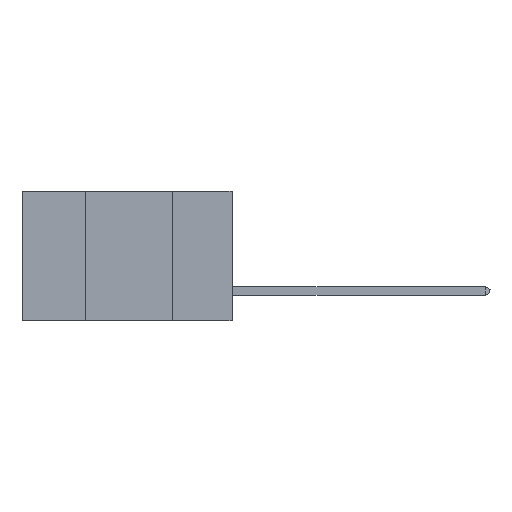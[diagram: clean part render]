
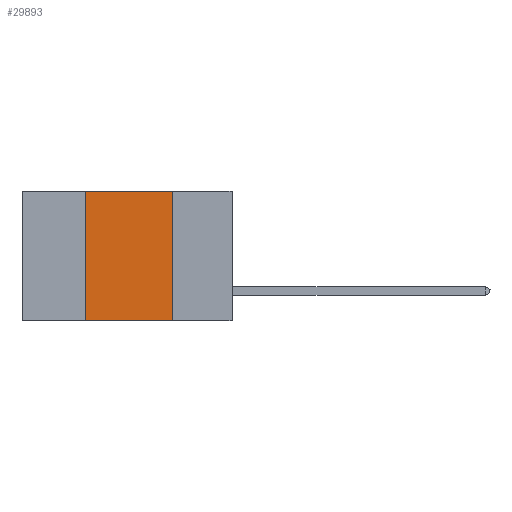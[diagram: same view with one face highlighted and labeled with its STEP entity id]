
A CAD part, left-side view. The second image highlights one B-rep face of the part: STEP entity #29893.
In plain terms, the highlighted planar face has unit normal (-1, 0, 0).
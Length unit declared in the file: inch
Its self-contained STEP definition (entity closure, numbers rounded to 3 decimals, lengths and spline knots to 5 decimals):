
#65 = EDGE_LOOP ( 'NONE', ( #20425, #28894, #29847, #20932 ) ) ;
#363 = EDGE_CURVE ( 'NONE', #22972, #16654, #29425, .T. ) ;
#664 = PLANE ( 'NONE',  #15403 ) ;
#749 = EDGE_CURVE ( 'NONE', #7456, #1954, #1974, .T. ) ;
#1749 = EDGE_CURVE ( 'NONE', #7456, #22972, #27541, .T. ) ;
#1954 = VERTEX_POINT ( 'NONE', #15884 ) ;
#1974 = LINE ( 'NONE', #10816, #25741 ) ;
#3836 = DIRECTION ( 'NONE',  ( 0., 0., 1. ) ) ;
#4505 = DIRECTION ( 'NONE',  ( 0., -1., 0. ) ) ;
#6804 = CARTESIAN_POINT ( 'NONE',  ( 0., 0.6, 0. ) ) ;
#7126 = LINE ( 'NONE', #12004, #9635 ) ;
#7456 = VERTEX_POINT ( 'NONE', #26695 ) ;
#8820 = DIRECTION ( 'NONE',  ( 0., -1., 0. ) ) ;
#9635 = VECTOR ( 'NONE', #14418, 39.37008 ) ;
#10238 = CARTESIAN_POINT ( 'NONE',  ( 0., 0.42, 0. ) ) ;
#10816 = CARTESIAN_POINT ( 'NONE',  ( 0., 0.6, -0.37 ) ) ;
#12004 = CARTESIAN_POINT ( 'NONE',  ( 0., 0.17, 0. ) ) ;
#14028 = EDGE_CURVE ( 'NONE', #16654, #1954, #7126, .T. ) ;
#14418 = DIRECTION ( 'NONE',  ( 0., 0., -1. ) ) ;
#15403 = AXIS2_PLACEMENT_3D ( 'NONE', #23320, #21112, #16593 ) ;
#15884 = CARTESIAN_POINT ( 'NONE',  ( 0., 0.17, -0.37 ) ) ;
#16593 = DIRECTION ( 'NONE',  ( 0., 0., -1. ) ) ;
#16654 = VERTEX_POINT ( 'NONE', #18955 ) ;
#17511 = VECTOR ( 'NONE', #4505, 39.37008 ) ;
#17647 = CARTESIAN_POINT ( 'NONE',  ( 0., 0.42, 0. ) ) ;
#18955 = CARTESIAN_POINT ( 'NONE',  ( 0., 0.17, 0. ) ) ;
#20425 = ORIENTED_EDGE ( 'NONE', *, *, #14028, .F. ) ;
#20932 = ORIENTED_EDGE ( 'NONE', *, *, #749, .T. ) ;
#21112 = DIRECTION ( 'NONE',  ( 1., 0., 0. ) ) ;
#22972 = VERTEX_POINT ( 'NONE', #10238 ) ;
#23320 = CARTESIAN_POINT ( 'NONE',  ( 0., 0.6, 0. ) ) ;
#23782 = FACE_OUTER_BOUND ( 'NONE', #65, .T. ) ;
#23875 = VECTOR ( 'NONE', #3836, 39.37008 ) ;
#25741 = VECTOR ( 'NONE', #8820, 39.37008 ) ;
#26695 = CARTESIAN_POINT ( 'NONE',  ( 0., 0.42, -0.37 ) ) ;
#27541 = LINE ( 'NONE', #17647, #23875 ) ;
#28894 = ORIENTED_EDGE ( 'NONE', *, *, #363, .F. ) ;
#29425 = LINE ( 'NONE', #6804, #17511 ) ;
#29847 = ORIENTED_EDGE ( 'NONE', *, *, #1749, .F. ) ;
#29893 = ADVANCED_FACE ( 'NONE', ( #23782 ), #664, .F. ) ;
